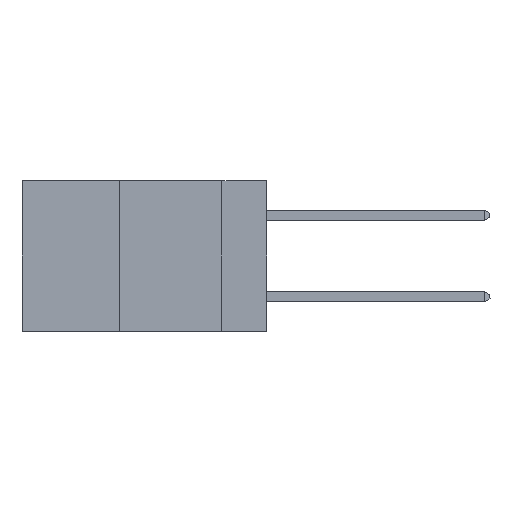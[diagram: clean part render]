
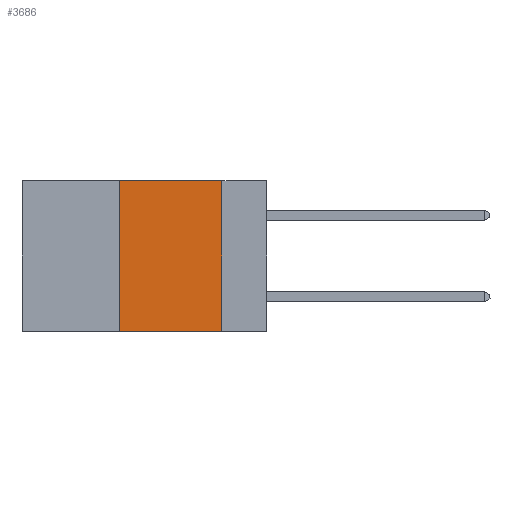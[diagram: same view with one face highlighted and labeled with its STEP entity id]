
A CAD part, left-side view. The second image highlights one B-rep face of the part: STEP entity #3686.
In plain terms, the highlighted planar face has unit normal (-1, 0, 0).
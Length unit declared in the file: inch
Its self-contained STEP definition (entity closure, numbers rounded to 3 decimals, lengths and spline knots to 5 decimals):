
#612 = DIRECTION ( 'NONE',  ( 0., -1., 0. ) ) ;
#1731 = DIRECTION ( 'NONE',  ( 0., -1., 0. ) ) ;
#1784 = ORIENTED_EDGE ( 'NONE', *, *, #6347, .F. ) ;
#2383 = LINE ( 'NONE', #18580, #17936 ) ;
#2469 = ORIENTED_EDGE ( 'NONE', *, *, #18900, .F. ) ;
#2823 = PLANE ( 'NONE',  #3282 ) ;
#3282 = AXIS2_PLACEMENT_3D ( 'NONE', #13294, #4264, #14884 ) ;
#3596 = ORIENTED_EDGE ( 'NONE', *, *, #5388, .F. ) ;
#3686 = ADVANCED_FACE ( 'NONE', ( #5823 ), #2823, .F. ) ;
#4264 = DIRECTION ( 'NONE',  ( 1., 0., 0. ) ) ;
#4411 = EDGE_CURVE ( 'NONE', #17058, #12469, #9009, .T. ) ;
#4513 = CARTESIAN_POINT ( 'NONE',  ( 0., 0.36, 0. ) ) ;
#4604 = LINE ( 'NONE', #17555, #8496 ) ;
#4670 = ORIENTED_EDGE ( 'NONE', *, *, #4411, .T. ) ;
#5388 = EDGE_CURVE ( 'NONE', #17058, #16704, #6927, .T. ) ;
#5501 = VERTEX_POINT ( 'NONE', #9252 ) ;
#5823 = FACE_OUTER_BOUND ( 'NONE', #13849, .T. ) ;
#6031 = CARTESIAN_POINT ( 'NONE',  ( 0., 0.36, 0. ) ) ;
#6347 = EDGE_CURVE ( 'NONE', #5501, #12469, #4604, .T. ) ;
#6927 = LINE ( 'NONE', #6031, #18660 ) ;
#8312 = DIRECTION ( 'NONE',  ( 0., 0., -1. ) ) ;
#8496 = VECTOR ( 'NONE', #8312, 39.37008 ) ;
#9009 = LINE ( 'NONE', #10505, #17245 ) ;
#9252 = CARTESIAN_POINT ( 'NONE',  ( 0., 0.11, 0. ) ) ;
#10505 = CARTESIAN_POINT ( 'NONE',  ( 0., 0.6, -0.37 ) ) ;
#12469 = VERTEX_POINT ( 'NONE', #19232 ) ;
#12699 = CARTESIAN_POINT ( 'NONE',  ( 0., 0.36, -0.37 ) ) ;
#13294 = CARTESIAN_POINT ( 'NONE',  ( 0., 0.6, 0. ) ) ;
#13647 = DIRECTION ( 'NONE',  ( 0., 0., 1. ) ) ;
#13849 = EDGE_LOOP ( 'NONE', ( #1784, #2469, #3596, #4670 ) ) ;
#14884 = DIRECTION ( 'NONE',  ( 0., 0., -1. ) ) ;
#16704 = VERTEX_POINT ( 'NONE', #4513 ) ;
#17058 = VERTEX_POINT ( 'NONE', #12699 ) ;
#17245 = VECTOR ( 'NONE', #1731, 39.37008 ) ;
#17555 = CARTESIAN_POINT ( 'NONE',  ( 0., 0.11, 0. ) ) ;
#17936 = VECTOR ( 'NONE', #612, 39.37008 ) ;
#18580 = CARTESIAN_POINT ( 'NONE',  ( 0., 0.6, 0. ) ) ;
#18660 = VECTOR ( 'NONE', #13647, 39.37008 ) ;
#18900 = EDGE_CURVE ( 'NONE', #16704, #5501, #2383, .T. ) ;
#19232 = CARTESIAN_POINT ( 'NONE',  ( 0., 0.11, -0.37 ) ) ;
